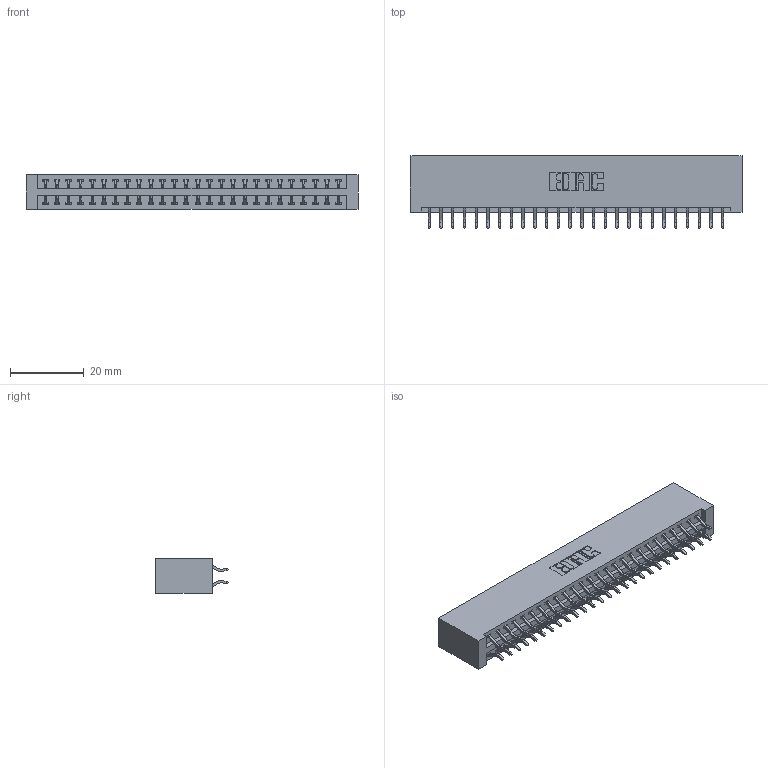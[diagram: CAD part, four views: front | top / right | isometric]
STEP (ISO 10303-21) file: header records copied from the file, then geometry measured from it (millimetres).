
FILE_DESCRIPTION (( 'STEP AP203' ), '1' );
FILE_NAME ('346-052-556-201.STEP', '2018-08-28T00:14:03', ( '' ), ( '' ), 'SwSTEP 2.0', 'SolidWorks 2016', '' );
FILE_SCHEMA (( 'CONFIG_CONTROL_DESIGN' ));
Length unit declared in the file: inch
Products named in the file (3): 346 Part_No Mounting Lugs; 345-292-001_556 Tail; 346-052-556-201
Assembly tree (53 placements, depth 2):
  346-052-556-201
    346 Part_No Mounting Lugs
    345-292-001_556 Tail  x52
Bounding box: 89.79 x 19.57 x 9.4 mm (x, y, z)
Volume: 9202.5 mm3; surface area: 12512.9 mm2
Topology: 53 solids, 53 shells, 3130 faces, 9301 edges, 6130 vertices
Faces by surface type: plane 2100, cylinder 1030
Entity records: 19065 total; most frequent: CARTESIAN_POINT 3176, ORIENTED_EDGE 3098, DIRECTION 2833, EDGE_CURVE 1549, LINE 1313, VECTOR 1313, VERTEX_POINT 1030, AXIS2_PLACEMENT_3D 760
